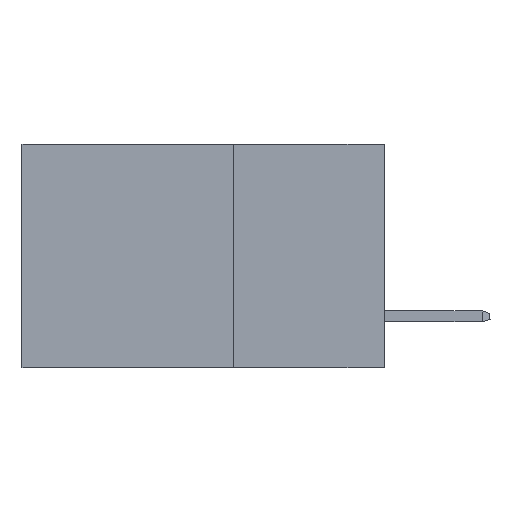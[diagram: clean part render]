
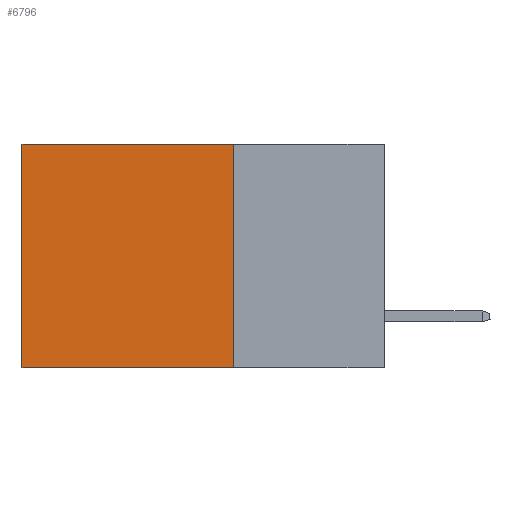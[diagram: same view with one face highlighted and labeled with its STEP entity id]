
A CAD part, left-side view. The second image highlights one B-rep face of the part: STEP entity #6796.
In plain terms, the highlighted planar face has unit normal (-1, 0, 0).
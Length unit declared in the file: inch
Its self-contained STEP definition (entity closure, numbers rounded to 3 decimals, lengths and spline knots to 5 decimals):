
#52 = EDGE_CURVE ( 'NONE', #8101, #12585, #7013, .T. ) ;
#603 = EDGE_CURVE ( 'NONE', #8901, #8101, #1991, .T. ) ;
#647 = LINE ( 'NONE', #2960, #2025 ) ;
#836 = ORIENTED_EDGE ( 'NONE', *, *, #10907, .T. ) ;
#880 = EDGE_LOOP ( 'NONE', ( #894, #11834, #3642, #836 ) ) ;
#886 = DIRECTION ( 'NONE',  ( 0., 1., 0. ) ) ;
#894 = ORIENTED_EDGE ( 'NONE', *, *, #3308, .T. ) ;
#999 = DIRECTION ( 'NONE',  ( 1., 0., 0. ) ) ;
#1171 = VECTOR ( 'NONE', #1188, 39.37008 ) ;
#1188 = DIRECTION ( 'NONE',  ( 0., 0., -1. ) ) ;
#1991 = LINE ( 'NONE', #12489, #9634 ) ;
#2025 = VECTOR ( 'NONE', #886, 39.37008 ) ;
#2053 = CARTESIAN_POINT ( 'NONE',  ( 0.298, 0.6, 0. ) ) ;
#2280 = CARTESIAN_POINT ( 'NONE',  ( 0.298, 0.25, -0.37 ) ) ;
#2901 = DIRECTION ( 'NONE',  ( 0., 0., -1. ) ) ;
#2960 = CARTESIAN_POINT ( 'NONE',  ( 0.298, 0.25, 0. ) ) ;
#3308 = EDGE_CURVE ( 'NONE', #9857, #12585, #6649, .T. ) ;
#3642 = ORIENTED_EDGE ( 'NONE', *, *, #603, .F. ) ;
#3924 = CARTESIAN_POINT ( 'NONE',  ( 0.298, 0.6, 0. ) ) ;
#3994 = PLANE ( 'NONE',  #12718 ) ;
#4385 = CARTESIAN_POINT ( 'NONE',  ( 0.298, 0.6, -0.37 ) ) ;
#5236 = CARTESIAN_POINT ( 'NONE',  ( 0.298, 0.25, -0.37 ) ) ;
#5590 = FACE_OUTER_BOUND ( 'NONE', #880, .T. ) ;
#6551 = DIRECTION ( 'NONE',  ( 0., 0., -1. ) ) ;
#6649 = LINE ( 'NONE', #2053, #1171 ) ;
#6796 = ADVANCED_FACE ( 'NONE', ( #5590 ), #3994, .F. ) ;
#7013 = LINE ( 'NONE', #2280, #8406 ) ;
#7437 = DIRECTION ( 'NONE',  ( 0., 1., 0. ) ) ;
#8101 = VERTEX_POINT ( 'NONE', #5236 ) ;
#8406 = VECTOR ( 'NONE', #7437, 39.37008 ) ;
#8571 = CARTESIAN_POINT ( 'NONE',  ( 0.298, 0.25, 0. ) ) ;
#8901 = VERTEX_POINT ( 'NONE', #8571 ) ;
#9634 = VECTOR ( 'NONE', #6551, 39.37008 ) ;
#9857 = VERTEX_POINT ( 'NONE', #3924 ) ;
#10907 = EDGE_CURVE ( 'NONE', #8901, #9857, #647, .T. ) ;
#11834 = ORIENTED_EDGE ( 'NONE', *, *, #52, .F. ) ;
#12031 = CARTESIAN_POINT ( 'NONE',  ( 0.298, 0.25, 0. ) ) ;
#12489 = CARTESIAN_POINT ( 'NONE',  ( 0.298, 0.25, 0. ) ) ;
#12585 = VERTEX_POINT ( 'NONE', #4385 ) ;
#12718 = AXIS2_PLACEMENT_3D ( 'NONE', #12031, #999, #2901 ) ;
